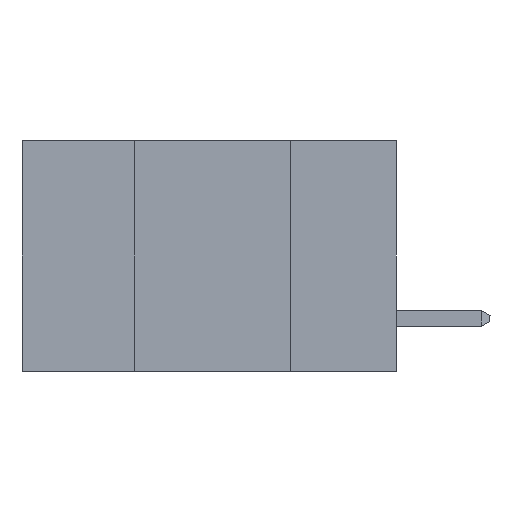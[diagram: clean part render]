
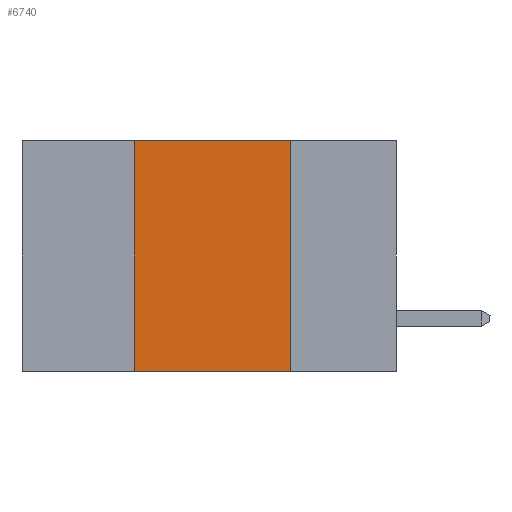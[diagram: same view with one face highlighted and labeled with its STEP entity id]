
A CAD part, left-side view. The second image highlights one B-rep face of the part: STEP entity #6740.
In plain terms, the highlighted planar face has unit normal (-1, 0, 0).
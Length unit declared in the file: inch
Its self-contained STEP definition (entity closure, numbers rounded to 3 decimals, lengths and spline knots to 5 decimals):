
#377 = ORIENTED_EDGE ( 'NONE', *, *, #10784, .T. ) ;
#437 = EDGE_LOOP ( 'NONE', ( #2043, #2899, #6021, #377 ) ) ;
#495 = VERTEX_POINT ( 'NONE', #3694 ) ;
#890 = DIRECTION ( 'NONE',  ( 0., -1., 0. ) ) ;
#1230 = VERTEX_POINT ( 'NONE', #3491 ) ;
#1845 = CARTESIAN_POINT ( 'NONE',  ( 0., 0.17, -0.37 ) ) ;
#2043 = ORIENTED_EDGE ( 'NONE', *, *, #2667, .F. ) ;
#2356 = VECTOR ( 'NONE', #9142, 39.37008 ) ;
#2483 = DIRECTION ( 'NONE',  ( 0., 0., 1. ) ) ;
#2647 = CARTESIAN_POINT ( 'NONE',  ( 0., 0.42, 0. ) ) ;
#2667 = EDGE_CURVE ( 'NONE', #495, #11084, #6424, .T. ) ;
#2703 = CARTESIAN_POINT ( 'NONE',  ( 0., 0.6, -0.37 ) ) ;
#2899 = ORIENTED_EDGE ( 'NONE', *, *, #5611, .F. ) ;
#3052 = LINE ( 'NONE', #6635, #10261 ) ;
#3491 = CARTESIAN_POINT ( 'NONE',  ( 0., 0.42, -0.37 ) ) ;
#3526 = LINE ( 'NONE', #2703, #3579 ) ;
#3579 = VECTOR ( 'NONE', #890, 39.37008 ) ;
#3694 = CARTESIAN_POINT ( 'NONE',  ( 0., 0.17, 0. ) ) ;
#4070 = VECTOR ( 'NONE', #2483, 39.37008 ) ;
#4542 = CARTESIAN_POINT ( 'NONE',  ( 0., 0.6, 0. ) ) ;
#5308 = EDGE_CURVE ( 'NONE', #1230, #9527, #8719, .T. ) ;
#5567 = AXIS2_PLACEMENT_3D ( 'NONE', #4542, #10712, #6284 ) ;
#5611 = EDGE_CURVE ( 'NONE', #9527, #495, #3052, .T. ) ;
#6021 = ORIENTED_EDGE ( 'NONE', *, *, #5308, .F. ) ;
#6284 = DIRECTION ( 'NONE',  ( 0., 0., -1. ) ) ;
#6424 = LINE ( 'NONE', #1845, #2356 ) ;
#6635 = CARTESIAN_POINT ( 'NONE',  ( 0., 0.6, 0. ) ) ;
#6740 = ADVANCED_FACE ( 'NONE', ( #7227 ), #10765, .F. ) ;
#7227 = FACE_OUTER_BOUND ( 'NONE', #437, .T. ) ;
#8653 = CARTESIAN_POINT ( 'NONE',  ( 0., 0.17, -0.37 ) ) ;
#8719 = LINE ( 'NONE', #9428, #4070 ) ;
#9142 = DIRECTION ( 'NONE',  ( 0., 0., -1. ) ) ;
#9428 = CARTESIAN_POINT ( 'NONE',  ( 0., 0.42, -0.37 ) ) ;
#9527 = VERTEX_POINT ( 'NONE', #2647 ) ;
#10225 = DIRECTION ( 'NONE',  ( 0., -1., 0. ) ) ;
#10261 = VECTOR ( 'NONE', #10225, 39.37008 ) ;
#10712 = DIRECTION ( 'NONE',  ( 1., 0., 0. ) ) ;
#10765 = PLANE ( 'NONE',  #5567 ) ;
#10784 = EDGE_CURVE ( 'NONE', #1230, #11084, #3526, .T. ) ;
#11084 = VERTEX_POINT ( 'NONE', #8653 ) ;
